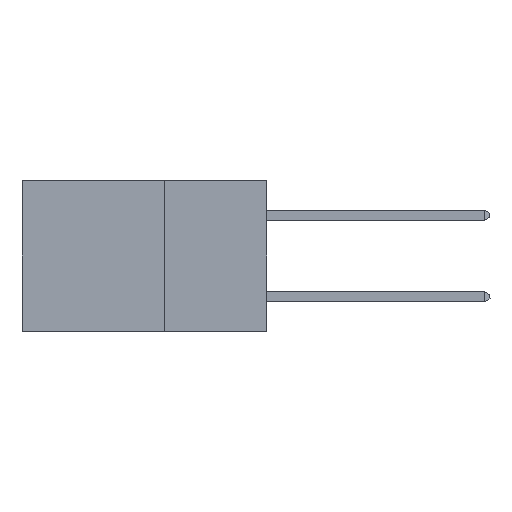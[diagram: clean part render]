
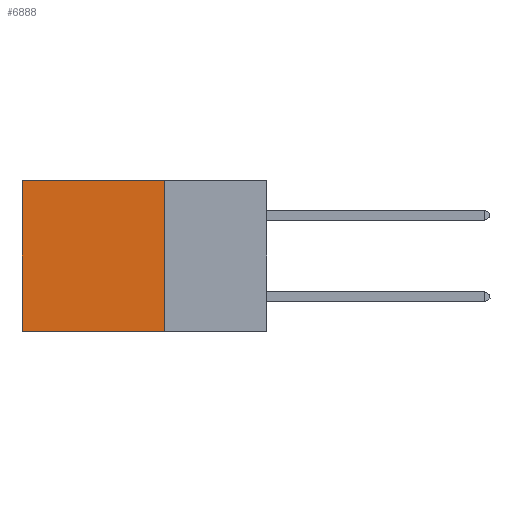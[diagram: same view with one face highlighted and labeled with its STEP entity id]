
A CAD part, left-side view. The second image highlights one B-rep face of the part: STEP entity #6888.
In plain terms, the highlighted planar face has unit normal (-1, 0, 0).
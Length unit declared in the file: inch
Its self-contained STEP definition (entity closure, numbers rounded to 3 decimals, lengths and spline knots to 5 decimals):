
#253 = LINE ( 'NONE', #15535, #13920 ) ;
#1234 = PLANE ( 'NONE',  #20463 ) ;
#1409 = CARTESIAN_POINT ( 'NONE',  ( 0.2875, 0.25, 0. ) ) ;
#1892 = CARTESIAN_POINT ( 'NONE',  ( 0.2875, 0.6, 0. ) ) ;
#2963 = DIRECTION ( 'NONE',  ( 0., 0., -1. ) ) ;
#3457 = VECTOR ( 'NONE', #16701, 39.37008 ) ;
#3654 = DIRECTION ( 'NONE',  ( 0., 1., 0. ) ) ;
#4182 = CARTESIAN_POINT ( 'NONE',  ( 0.2875, 0.25, 0. ) ) ;
#4606 = VERTEX_POINT ( 'NONE', #20894 ) ;
#5049 = EDGE_CURVE ( 'NONE', #4606, #8374, #6462, .T. ) ;
#5301 = ORIENTED_EDGE ( 'NONE', *, *, #5049, .T. ) ;
#5346 = ORIENTED_EDGE ( 'NONE', *, *, #17736, .F. ) ;
#5560 = ORIENTED_EDGE ( 'NONE', *, *, #8153, .F. ) ;
#5644 = ORIENTED_EDGE ( 'NONE', *, *, #6383, .T. ) ;
#6383 = EDGE_CURVE ( 'NONE', #8558, #4606, #253, .T. ) ;
#6462 = LINE ( 'NONE', #1892, #20914 ) ;
#6888 = ADVANCED_FACE ( 'NONE', ( #12314 ), #1234, .F. ) ;
#6933 = DIRECTION ( 'NONE',  ( 0., 1., 0. ) ) ;
#8153 = EDGE_CURVE ( 'NONE', #8558, #10335, #21286, .T. ) ;
#8374 = VERTEX_POINT ( 'NONE', #15631 ) ;
#8521 = EDGE_LOOP ( 'NONE', ( #5301, #5346, #5560, #5644 ) ) ;
#8558 = VERTEX_POINT ( 'NONE', #4182 ) ;
#9524 = VECTOR ( 'NONE', #6933, 39.37008 ) ;
#10335 = VERTEX_POINT ( 'NONE', #13802 ) ;
#10439 = DIRECTION ( 'NONE',  ( 0., 0., -1. ) ) ;
#11519 = CARTESIAN_POINT ( 'NONE',  ( 0.2875, 0.25, 0. ) ) ;
#12314 = FACE_OUTER_BOUND ( 'NONE', #8521, .T. ) ;
#13203 = DIRECTION ( 'NONE',  ( 1., 0., 0. ) ) ;
#13802 = CARTESIAN_POINT ( 'NONE',  ( 0.2875, 0.25, -0.37 ) ) ;
#13920 = VECTOR ( 'NONE', #3654, 39.37008 ) ;
#15429 = CARTESIAN_POINT ( 'NONE',  ( 0.2875, 0.25, -0.37 ) ) ;
#15535 = CARTESIAN_POINT ( 'NONE',  ( 0.2875, 0.25, 0. ) ) ;
#15631 = CARTESIAN_POINT ( 'NONE',  ( 0.2875, 0.6, -0.37 ) ) ;
#16701 = DIRECTION ( 'NONE',  ( 0., 0., -1. ) ) ;
#17736 = EDGE_CURVE ( 'NONE', #10335, #8374, #17909, .T. ) ;
#17909 = LINE ( 'NONE', #15429, #9524 ) ;
#20463 = AXIS2_PLACEMENT_3D ( 'NONE', #11519, #13203, #2963 ) ;
#20894 = CARTESIAN_POINT ( 'NONE',  ( 0.2875, 0.6, 0. ) ) ;
#20914 = VECTOR ( 'NONE', #10439, 39.37008 ) ;
#21286 = LINE ( 'NONE', #1409, #3457 ) ;
